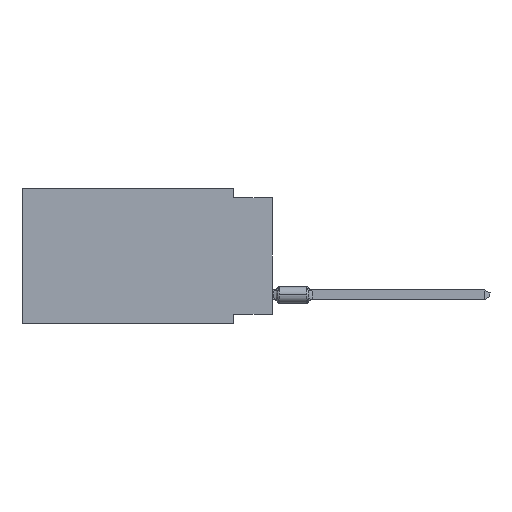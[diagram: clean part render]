
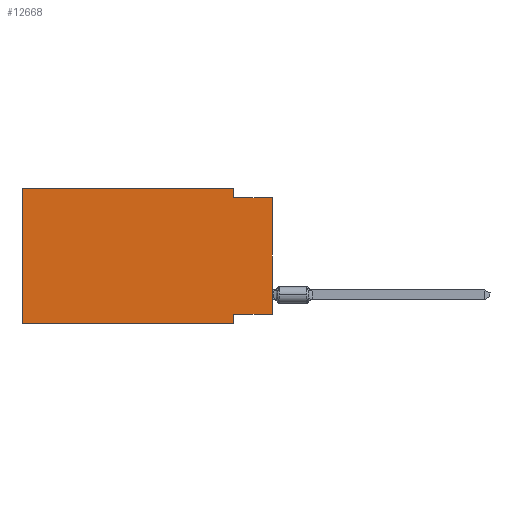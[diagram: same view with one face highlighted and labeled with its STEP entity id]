
A CAD part, left-side view. The second image highlights one B-rep face of the part: STEP entity #12668.
In plain terms, the highlighted planar face has unit normal (-1, 0, 0).
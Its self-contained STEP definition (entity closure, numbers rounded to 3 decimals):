
#1146 = CARTESIAN_POINT ( 'NONE',  ( 0., 2.54, -0.635 ) ) ;
#2066 = VERTEX_POINT ( 'NONE', #18764 ) ;
#2258 = EDGE_CURVE ( 'NONE', #2066, #46908, #53643, .T. ) ;
#3519 = EDGE_CURVE ( 'NONE', #36570, #23141, #19695, .T. ) ;
#4392 = DIRECTION ( 'NONE',  ( 0., 0., -1. ) ) ;
#5034 = CARTESIAN_POINT ( 'NONE',  ( 0., 16.383, -8.89 ) ) ;
#5138 = EDGE_LOOP ( 'NONE', ( #36932, #36257, #6433, #30472, #47980, #12308, #56771, #55478 ) ) ;
#5299 = VECTOR ( 'NONE', #22521, 1000. ) ;
#5526 = EDGE_CURVE ( 'NONE', #38788, #10797, #10425, .T. ) ;
#6433 = ORIENTED_EDGE ( 'NONE', *, *, #15531, .F. ) ;
#7405 = EDGE_CURVE ( 'NONE', #10797, #46908, #44516, .T. ) ;
#8711 = CARTESIAN_POINT ( 'NONE',  ( 0., 2.54, 0. ) ) ;
#10080 = CARTESIAN_POINT ( 'NONE',  ( 0., 2.54, -8.89 ) ) ;
#10425 = LINE ( 'NONE', #41095, #17095 ) ;
#10797 = VERTEX_POINT ( 'NONE', #51874 ) ;
#11716 = DIRECTION ( 'NONE',  ( 1., 0., 0. ) ) ;
#12284 = DIRECTION ( 'NONE',  ( 0., 0., -1. ) ) ;
#12308 = ORIENTED_EDGE ( 'NONE', *, *, #2258, .T. ) ;
#12668 = ADVANCED_FACE ( 'NONE', ( #25315 ), #21554, .F. ) ;
#12983 = VERTEX_POINT ( 'NONE', #43548 ) ;
#15531 = EDGE_CURVE ( 'NONE', #43755, #36570, #35332, .T. ) ;
#16974 = CARTESIAN_POINT ( 'NONE',  ( 0., 0., -8.255 ) ) ;
#17095 = VECTOR ( 'NONE', #32422, 1000. ) ;
#18276 = EDGE_CURVE ( 'NONE', #12983, #43755, #32920, .T. ) ;
#18638 = DIRECTION ( 'NONE',  ( 0., -1., 0. ) ) ;
#18764 = CARTESIAN_POINT ( 'NONE',  ( 0., 16.383, -8.89 ) ) ;
#18837 = DIRECTION ( 'NONE',  ( 0., -1., 0. ) ) ;
#19695 = LINE ( 'NONE', #41096, #36396 ) ;
#19867 = DIRECTION ( 'NONE',  ( 0., 0., 1. ) ) ;
#20260 = CARTESIAN_POINT ( 'NONE',  ( 0., 2.54, -8.89 ) ) ;
#21193 = VECTOR ( 'NONE', #33470, 1000. ) ;
#21554 = PLANE ( 'NONE',  #53124 ) ;
#22521 = DIRECTION ( 'NONE',  ( 0., 0., -1. ) ) ;
#23068 = EDGE_CURVE ( 'NONE', #2066, #12983, #54663, .T. ) ;
#23141 = VERTEX_POINT ( 'NONE', #29401 ) ;
#25313 = CARTESIAN_POINT ( 'NONE',  ( 0., 0., 0. ) ) ;
#25315 = FACE_OUTER_BOUND ( 'NONE', #5138, .T. ) ;
#25557 = VECTOR ( 'NONE', #4392, 1000. ) ;
#29401 = CARTESIAN_POINT ( 'NONE',  ( 0., 0., -0.635 ) ) ;
#30472 = ORIENTED_EDGE ( 'NONE', *, *, #18276, .F. ) ;
#32422 = DIRECTION ( 'NONE',  ( 0., 1., 0. ) ) ;
#32912 = CARTESIAN_POINT ( 'NONE',  ( 0., 16.383, 0. ) ) ;
#32920 = LINE ( 'NONE', #38092, #21193 ) ;
#33470 = DIRECTION ( 'NONE',  ( 0., -1., 0. ) ) ;
#33737 = DIRECTION ( 'NONE',  ( 0., 0., 1. ) ) ;
#35332 = LINE ( 'NONE', #8711, #25557 ) ;
#36257 = ORIENTED_EDGE ( 'NONE', *, *, #3519, .F. ) ;
#36396 = VECTOR ( 'NONE', #18837, 1000. ) ;
#36570 = VERTEX_POINT ( 'NONE', #1146 ) ;
#36833 = VECTOR ( 'NONE', #19867, 1000. ) ;
#36932 = ORIENTED_EDGE ( 'NONE', *, *, #37409, .T. ) ;
#37409 = EDGE_CURVE ( 'NONE', #38788, #23141, #46195, .T. ) ;
#38092 = CARTESIAN_POINT ( 'NONE',  ( 0., 16.383, 0. ) ) ;
#38788 = VERTEX_POINT ( 'NONE', #16974 ) ;
#41095 = CARTESIAN_POINT ( 'NONE',  ( 0., 0., -8.255 ) ) ;
#41096 = CARTESIAN_POINT ( 'NONE',  ( 0., 0., -0.635 ) ) ;
#41964 = CARTESIAN_POINT ( 'NONE',  ( 0., 2.54, 0. ) ) ;
#43548 = CARTESIAN_POINT ( 'NONE',  ( 0., 16.383, 0. ) ) ;
#43755 = VERTEX_POINT ( 'NONE', #41964 ) ;
#44516 = LINE ( 'NONE', #10080, #5299 ) ;
#46195 = LINE ( 'NONE', #25313, #36833 ) ;
#46908 = VERTEX_POINT ( 'NONE', #20260 ) ;
#47372 = VECTOR ( 'NONE', #33737, 1000. ) ;
#47581 = CARTESIAN_POINT ( 'NONE',  ( 0., 16.383, 0. ) ) ;
#47980 = ORIENTED_EDGE ( 'NONE', *, *, #23068, .F. ) ;
#51874 = CARTESIAN_POINT ( 'NONE',  ( 0., 2.54, -8.255 ) ) ;
#53124 = AXIS2_PLACEMENT_3D ( 'NONE', #47581, #11716, #12284 ) ;
#53643 = LINE ( 'NONE', #5034, #55655 ) ;
#54663 = LINE ( 'NONE', #32912, #47372 ) ;
#55478 = ORIENTED_EDGE ( 'NONE', *, *, #5526, .F. ) ;
#55655 = VECTOR ( 'NONE', #18638, 1000. ) ;
#56771 = ORIENTED_EDGE ( 'NONE', *, *, #7405, .F. ) ;
